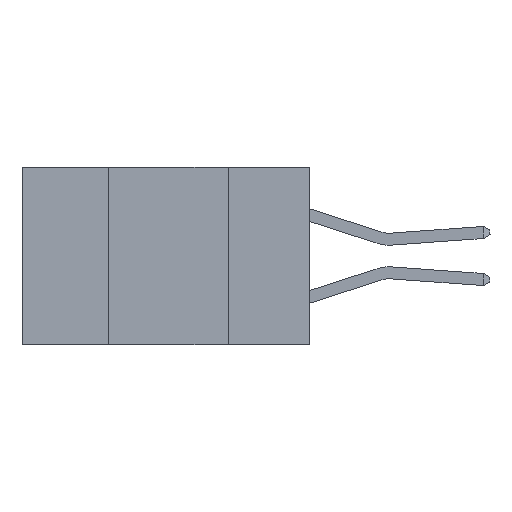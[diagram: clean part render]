
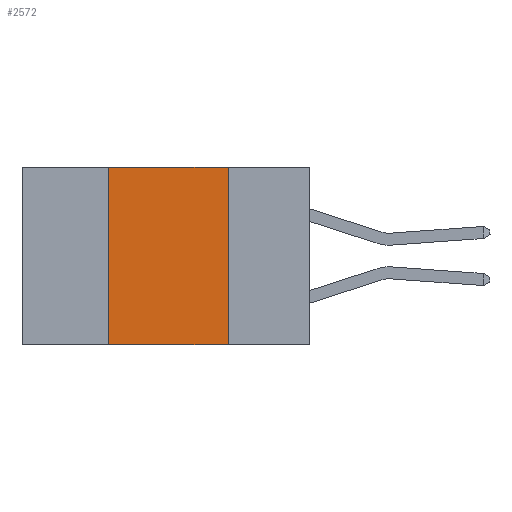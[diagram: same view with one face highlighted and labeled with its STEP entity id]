
A CAD part, left-side view. The second image highlights one B-rep face of the part: STEP entity #2572.
In plain terms, the highlighted planar face has unit normal (-1, 0, 0).
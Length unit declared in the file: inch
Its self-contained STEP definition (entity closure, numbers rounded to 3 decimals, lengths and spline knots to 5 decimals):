
#18 = VERTEX_POINT ( 'NONE', #5350 ) ;
#70 = CARTESIAN_POINT ( 'NONE',  ( 0., 0.42, 0. ) ) ;
#222 = DIRECTION ( 'NONE',  ( 0., 0., 1. ) ) ;
#238 = VECTOR ( 'NONE', #485, 39.37008 ) ;
#292 = AXIS2_PLACEMENT_3D ( 'NONE', #4890, #2347, #8237 ) ;
#485 = DIRECTION ( 'NONE',  ( 0., 0., -1. ) ) ;
#618 = PLANE ( 'NONE',  #292 ) ;
#1082 = DIRECTION ( 'NONE',  ( 0., -1., 0. ) ) ;
#1249 = EDGE_LOOP ( 'NONE', ( #9936, #10799, #8785, #5722 ) ) ;
#1281 = CARTESIAN_POINT ( 'NONE',  ( 0., 0.17, 0. ) ) ;
#1837 = EDGE_CURVE ( 'NONE', #5130, #6126, #4032, .T. ) ;
#2347 = DIRECTION ( 'NONE',  ( 1., 0., 0. ) ) ;
#2572 = ADVANCED_FACE ( 'NONE', ( #10555 ), #618, .F. ) ;
#2573 = VERTEX_POINT ( 'NONE', #3852 ) ;
#3852 = CARTESIAN_POINT ( 'NONE',  ( 0., 0.42, 0. ) ) ;
#3976 = EDGE_CURVE ( 'NONE', #18, #6126, #10256, .T. ) ;
#4032 = LINE ( 'NONE', #8830, #238 ) ;
#4405 = CARTESIAN_POINT ( 'NONE',  ( 0., 0.6, -0.37 ) ) ;
#4890 = CARTESIAN_POINT ( 'NONE',  ( 0., 0.6, 0. ) ) ;
#5130 = VERTEX_POINT ( 'NONE', #1281 ) ;
#5350 = CARTESIAN_POINT ( 'NONE',  ( 0., 0.42, -0.37 ) ) ;
#5722 = ORIENTED_EDGE ( 'NONE', *, *, #3976, .T. ) ;
#6069 = VECTOR ( 'NONE', #222, 39.37008 ) ;
#6126 = VERTEX_POINT ( 'NONE', #9249 ) ;
#6743 = VECTOR ( 'NONE', #1082, 39.37008 ) ;
#7219 = EDGE_CURVE ( 'NONE', #2573, #5130, #8580, .T. ) ;
#8237 = DIRECTION ( 'NONE',  ( 0., 0., -1. ) ) ;
#8534 = EDGE_CURVE ( 'NONE', #18, #2573, #9973, .T. ) ;
#8580 = LINE ( 'NONE', #10140, #8692 ) ;
#8692 = VECTOR ( 'NONE', #9375, 39.37008 ) ;
#8785 = ORIENTED_EDGE ( 'NONE', *, *, #8534, .F. ) ;
#8830 = CARTESIAN_POINT ( 'NONE',  ( 0., 0.17, 0. ) ) ;
#9249 = CARTESIAN_POINT ( 'NONE',  ( 0., 0.17, -0.37 ) ) ;
#9375 = DIRECTION ( 'NONE',  ( 0., -1., 0. ) ) ;
#9936 = ORIENTED_EDGE ( 'NONE', *, *, #1837, .F. ) ;
#9973 = LINE ( 'NONE', #70, #6069 ) ;
#10140 = CARTESIAN_POINT ( 'NONE',  ( 0., 0.6, 0. ) ) ;
#10256 = LINE ( 'NONE', #4405, #6743 ) ;
#10555 = FACE_OUTER_BOUND ( 'NONE', #1249, .T. ) ;
#10799 = ORIENTED_EDGE ( 'NONE', *, *, #7219, .F. ) ;
